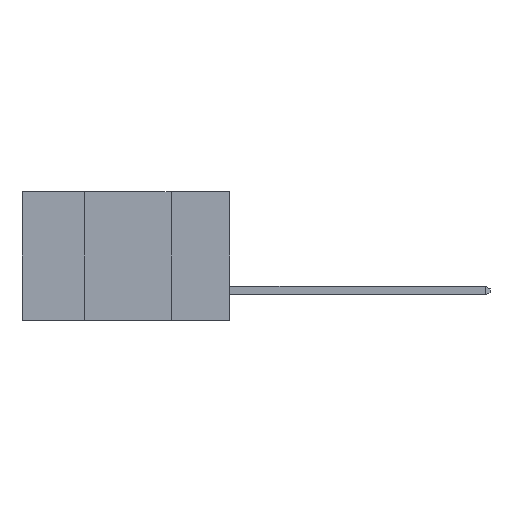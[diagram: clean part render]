
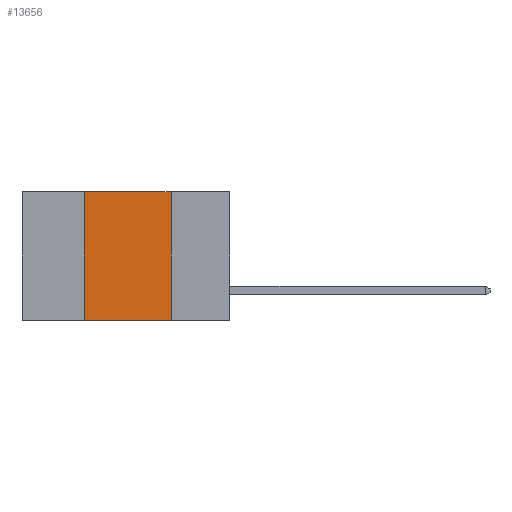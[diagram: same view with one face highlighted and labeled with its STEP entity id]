
A CAD part, left-side view. The second image highlights one B-rep face of the part: STEP entity #13656.
In plain terms, the highlighted planar face has unit normal (-1, 0, 0).
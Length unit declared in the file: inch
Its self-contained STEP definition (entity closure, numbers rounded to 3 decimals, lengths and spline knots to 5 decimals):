
#106 = EDGE_CURVE ( 'NONE', #142, #1185, #12336, .T. ) ;
#135 = ORIENTED_EDGE ( 'NONE', *, *, #11135, .F. ) ;
#142 = VERTEX_POINT ( 'NONE', #3034 ) ;
#235 = ORIENTED_EDGE ( 'NONE', *, *, #4905, .F. ) ;
#251 = ORIENTED_EDGE ( 'NONE', *, *, #106, .F. ) ;
#346 = ORIENTED_EDGE ( 'NONE', *, *, #10648, .T. ) ;
#1185 = VERTEX_POINT ( 'NONE', #5163 ) ;
#1708 = EDGE_LOOP ( 'NONE', ( #135, #235, #251, #346 ) ) ;
#2610 = VERTEX_POINT ( 'NONE', #7660 ) ;
#2642 = VECTOR ( 'NONE', #10276, 39.37008 ) ;
#3034 = CARTESIAN_POINT ( 'NONE',  ( 0., 0.42, -0.37 ) ) ;
#3212 = VERTEX_POINT ( 'NONE', #5953 ) ;
#4871 = DIRECTION ( 'NONE',  ( 0., -1., 0. ) ) ;
#4905 = EDGE_CURVE ( 'NONE', #1185, #2610, #11574, .T. ) ;
#5163 = CARTESIAN_POINT ( 'NONE',  ( 0., 0.42, 0. ) ) ;
#5444 = DIRECTION ( 'NONE',  ( 1., 0., 0. ) ) ;
#5953 = CARTESIAN_POINT ( 'NONE',  ( 0., 0.17, -0.37 ) ) ;
#7340 = CARTESIAN_POINT ( 'NONE',  ( 0., 0.17, 0. ) ) ;
#7660 = CARTESIAN_POINT ( 'NONE',  ( 0., 0.17, 0. ) ) ;
#7862 = AXIS2_PLACEMENT_3D ( 'NONE', #8945, #5444, #13739 ) ;
#8532 = DIRECTION ( 'NONE',  ( 0., 0., -1. ) ) ;
#8579 = LINE ( 'NONE', #7340, #14518 ) ;
#8597 = CARTESIAN_POINT ( 'NONE',  ( 0., 0.6, -0.37 ) ) ;
#8796 = VECTOR ( 'NONE', #9788, 39.37008 ) ;
#8945 = CARTESIAN_POINT ( 'NONE',  ( 0., 0.6, 0. ) ) ;
#9575 = CARTESIAN_POINT ( 'NONE',  ( 0., 0.6, 0. ) ) ;
#9788 = DIRECTION ( 'NONE',  ( 0., -1., 0. ) ) ;
#10182 = CARTESIAN_POINT ( 'NONE',  ( 0., 0.42, 0. ) ) ;
#10276 = DIRECTION ( 'NONE',  ( 0., 0., 1. ) ) ;
#10648 = EDGE_CURVE ( 'NONE', #142, #3212, #12335, .T. ) ;
#10764 = FACE_OUTER_BOUND ( 'NONE', #1708, .T. ) ;
#11135 = EDGE_CURVE ( 'NONE', #2610, #3212, #8579, .T. ) ;
#11574 = LINE ( 'NONE', #9575, #14689 ) ;
#12335 = LINE ( 'NONE', #8597, #8796 ) ;
#12336 = LINE ( 'NONE', #10182, #2642 ) ;
#12594 = PLANE ( 'NONE',  #7862 ) ;
#13656 = ADVANCED_FACE ( 'NONE', ( #10764 ), #12594, .F. ) ;
#13739 = DIRECTION ( 'NONE',  ( 0., 0., -1. ) ) ;
#14518 = VECTOR ( 'NONE', #8532, 39.37008 ) ;
#14689 = VECTOR ( 'NONE', #4871, 39.37008 ) ;
